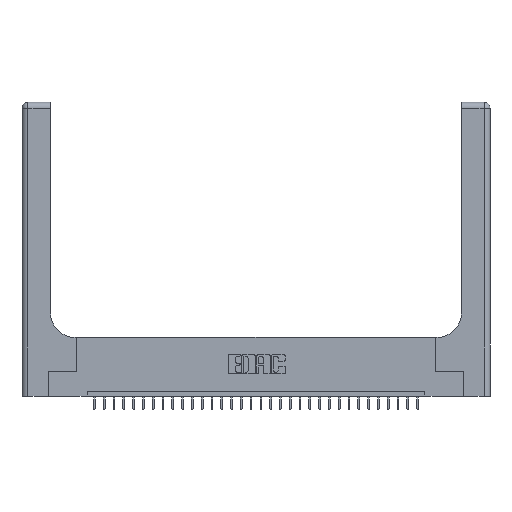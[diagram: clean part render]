
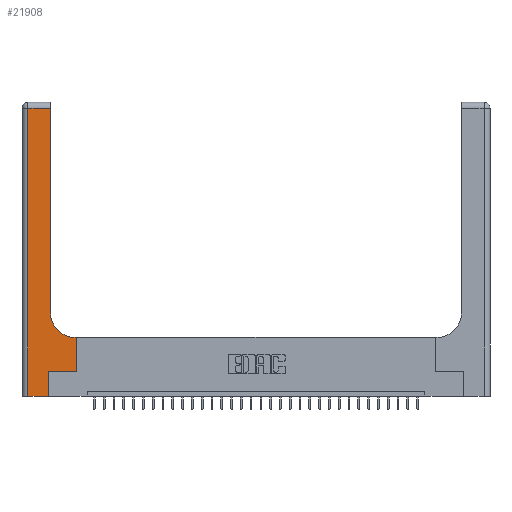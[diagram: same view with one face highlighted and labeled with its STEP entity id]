
A CAD part, top view. The second image highlights one B-rep face of the part: STEP entity #21908.
In plain terms, the highlighted planar face has unit normal (0, 0, 1).
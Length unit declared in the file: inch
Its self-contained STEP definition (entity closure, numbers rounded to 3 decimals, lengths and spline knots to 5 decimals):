
#609 = VERTEX_POINT ( 'NONE', #7808 ) ;
#907 = EDGE_CURVE ( 'NONE', #21585, #4006, #22482, .T. ) ;
#1462 = LINE ( 'NONE', #18923, #14045 ) ;
#1520 = VERTEX_POINT ( 'NONE', #28407 ) ;
#1597 = EDGE_CURVE ( 'NONE', #20444, #12261, #27830, .T. ) ;
#2331 = ORIENTED_EDGE ( 'NONE', *, *, #24147, .T. ) ;
#2455 = ORIENTED_EDGE ( 'NONE', *, *, #27562, .T. ) ;
#2522 = CARTESIAN_POINT ( 'NONE',  ( 0.2915, 3., 0.37 ) ) ;
#2552 = CARTESIAN_POINT ( 'NONE',  ( 0., 3., 0.37 ) ) ;
#2773 = ORIENTED_EDGE ( 'NONE', *, *, #25367, .T. ) ;
#2870 = FACE_OUTER_BOUND ( 'NONE', #17455, .T. ) ;
#2925 = DIRECTION ( 'NONE',  ( 0., -1., 0. ) ) ;
#3368 = VECTOR ( 'NONE', #31751, 39.37008 ) ;
#3456 = VECTOR ( 'NONE', #17588, 39.37008 ) ;
#3704 = VECTOR ( 'NONE', #29445, 39.37008 ) ;
#3710 = CARTESIAN_POINT ( 'NONE',  ( 0.5415, 0.6, 0.37 ) ) ;
#4006 = VERTEX_POINT ( 'NONE', #31428 ) ;
#4214 = CARTESIAN_POINT ( 'NONE',  ( 0.2915, 0.6, 0.37 ) ) ;
#4568 = ORIENTED_EDGE ( 'NONE', *, *, #25154, .T. ) ;
#4611 = VECTOR ( 'NONE', #21907, 39.37008 ) ;
#4612 = LINE ( 'NONE', #12035, #4611 ) ;
#6901 = ORIENTED_EDGE ( 'NONE', *, *, #1597, .T. ) ;
#7499 = ORIENTED_EDGE ( 'NONE', *, *, #22393, .T. ) ;
#7748 = VECTOR ( 'NONE', #23328, 39.37008 ) ;
#7808 = CARTESIAN_POINT ( 'NONE',  ( 0.269, 0., 0.37 ) ) ;
#9972 = DIRECTION ( 'NONE',  ( -1., 0., 0. ) ) ;
#11309 = DIRECTION ( 'NONE',  ( 0., 1., 0. ) ) ;
#11512 = LINE ( 'NONE', #14098, #7748 ) ;
#11869 = CARTESIAN_POINT ( 'NONE',  ( 0.5585, 0.6, 0.37 ) ) ;
#12035 = CARTESIAN_POINT ( 'NONE',  ( 0., 0., 0.37 ) ) ;
#12261 = VERTEX_POINT ( 'NONE', #22638 ) ;
#12868 = DIRECTION ( 'NONE',  ( 0., 0., -1. ) ) ;
#13845 = DIRECTION ( 'NONE',  ( 1., 0., 0. ) ) ;
#13878 = AXIS2_PLACEMENT_3D ( 'NONE', #30496, #18235, #13845 ) ;
#14045 = VECTOR ( 'NONE', #11309, 39.37008 ) ;
#14098 = CARTESIAN_POINT ( 'NONE',  ( 0., 2.94, 0.37 ) ) ;
#15016 = ORIENTED_EDGE ( 'NONE', *, *, #17810, .T. ) ;
#15369 = EDGE_CURVE ( 'NONE', #12261, #1520, #24648, .T. ) ;
#15578 = VERTEX_POINT ( 'NONE', #23194 ) ;
#17455 = EDGE_LOOP ( 'NONE', ( #21788, #2455, #22001, #7499, #15016, #4568, #2773, #2331, #6901 ) ) ;
#17588 = DIRECTION ( 'NONE',  ( 0., 1., 0. ) ) ;
#17810 = EDGE_CURVE ( 'NONE', #609, #21595, #24867, .T. ) ;
#18235 = DIRECTION ( 'NONE',  ( 0., 0., -1. ) ) ;
#18622 = VECTOR ( 'NONE', #31327, 39.37008 ) ;
#18923 = CARTESIAN_POINT ( 'NONE',  ( 0.5585, 0.25, 0.37 ) ) ;
#19449 = CARTESIAN_POINT ( 'NONE',  ( 0.06, 2.94, 0.37 ) ) ;
#20182 = CARTESIAN_POINT ( 'NONE',  ( 0.269, 0., 0.37 ) ) ;
#20444 = VERTEX_POINT ( 'NONE', #3710 ) ;
#21585 = VERTEX_POINT ( 'NONE', #19449 ) ;
#21595 = VERTEX_POINT ( 'NONE', #29292 ) ;
#21788 = ORIENTED_EDGE ( 'NONE', *, *, #15369, .T. ) ;
#21907 = DIRECTION ( 'NONE',  ( 1., 0., 0. ) ) ;
#21908 = ADVANCED_FACE ( 'NONE', ( #2870 ), #31782, .F. ) ;
#22001 = ORIENTED_EDGE ( 'NONE', *, *, #907, .T. ) ;
#22185 = VERTEX_POINT ( 'NONE', #11869 ) ;
#22393 = EDGE_CURVE ( 'NONE', #4006, #609, #4612, .T. ) ;
#22482 = LINE ( 'NONE', #27499, #23671 ) ;
#22638 = CARTESIAN_POINT ( 'NONE',  ( 0.2915, 0.85, 0.37 ) ) ;
#23194 = CARTESIAN_POINT ( 'NONE',  ( 0.5585, 0.25, 0.37 ) ) ;
#23328 = DIRECTION ( 'NONE',  ( -1., 0., 0. ) ) ;
#23671 = VECTOR ( 'NONE', #2925, 39.37008 ) ;
#24147 = EDGE_CURVE ( 'NONE', #22185, #20444, #26353, .T. ) ;
#24440 = LINE ( 'NONE', #27040, #3704 ) ;
#24648 = LINE ( 'NONE', #2522, #3368 ) ;
#24867 = LINE ( 'NONE', #20182, #3456 ) ;
#25154 = EDGE_CURVE ( 'NONE', #21595, #15578, #24440, .T. ) ;
#25367 = EDGE_CURVE ( 'NONE', #15578, #22185, #1462, .T. ) ;
#26353 = LINE ( 'NONE', #4214, #18622 ) ;
#27040 = CARTESIAN_POINT ( 'NONE',  ( 0.269, 0.25, 0.37 ) ) ;
#27499 = CARTESIAN_POINT ( 'NONE',  ( 0.06, 3., 0.37 ) ) ;
#27562 = EDGE_CURVE ( 'NONE', #1520, #21585, #11512, .T. ) ;
#27830 = CIRCLE ( 'NONE', #13878, 0.25 ) ;
#28407 = CARTESIAN_POINT ( 'NONE',  ( 0.2915, 2.94, 0.37 ) ) ;
#29292 = CARTESIAN_POINT ( 'NONE',  ( 0.269, 0.25, 0.37 ) ) ;
#29445 = DIRECTION ( 'NONE',  ( 1., 0., 0. ) ) ;
#30496 = CARTESIAN_POINT ( 'NONE',  ( 0.5415, 0.85, 0.37 ) ) ;
#31327 = DIRECTION ( 'NONE',  ( -1., 0., 0. ) ) ;
#31428 = CARTESIAN_POINT ( 'NONE',  ( 0.06, 0., 0.37 ) ) ;
#31751 = DIRECTION ( 'NONE',  ( 0., 1., 0. ) ) ;
#31782 = PLANE ( 'NONE',  #31909 ) ;
#31909 = AXIS2_PLACEMENT_3D ( 'NONE', #2552, #12868, #9972 ) ;
